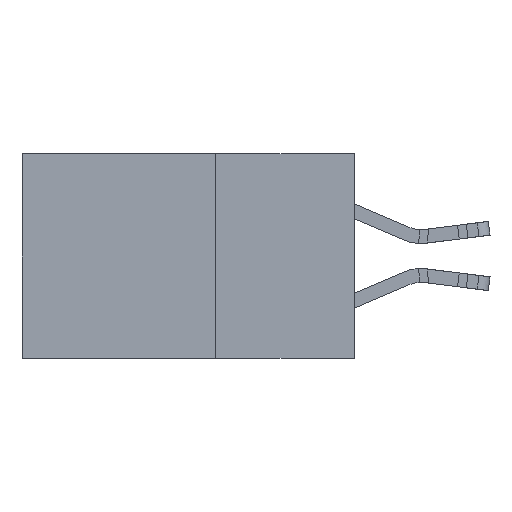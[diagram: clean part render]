
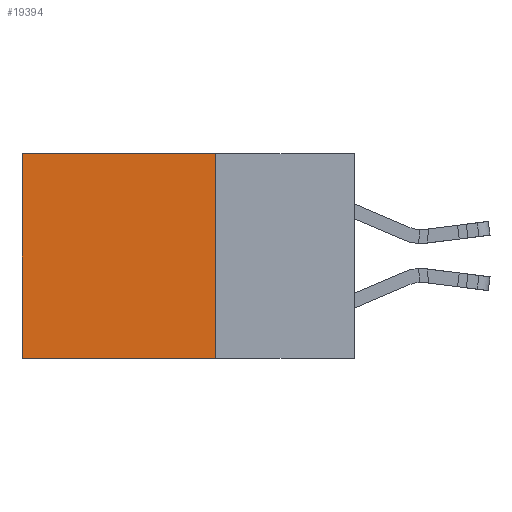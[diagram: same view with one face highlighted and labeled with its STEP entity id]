
A CAD part, left-side view. The second image highlights one B-rep face of the part: STEP entity #19394.
In plain terms, the highlighted planar face has unit normal (-1, 0, 0).
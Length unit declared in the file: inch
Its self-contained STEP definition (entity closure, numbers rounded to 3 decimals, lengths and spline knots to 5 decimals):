
#275 = LINE ( 'NONE', #14982, #15777 ) ;
#353 = ORIENTED_EDGE ( 'NONE', *, *, #2077, .T. ) ;
#1953 = ORIENTED_EDGE ( 'NONE', *, *, #19476, .F. ) ;
#2077 = EDGE_CURVE ( 'NONE', #3787, #19937, #25806, .T. ) ;
#2688 = CARTESIAN_POINT ( 'NONE',  ( 0.2615, 0.6, -0.37 ) ) ;
#3787 = VERTEX_POINT ( 'NONE', #11315 ) ;
#4360 = CARTESIAN_POINT ( 'NONE',  ( 0.2615, 0.25, 0. ) ) ;
#5278 = PLANE ( 'NONE',  #10027 ) ;
#6476 = CARTESIAN_POINT ( 'NONE',  ( 0.2615, 0.6, -0.37 ) ) ;
#6988 = ORIENTED_EDGE ( 'NONE', *, *, #23556, .F. ) ;
#7903 = DIRECTION ( 'NONE',  ( 0., 0., -1. ) ) ;
#8521 = DIRECTION ( 'NONE',  ( 0., 0., -1. ) ) ;
#10027 = AXIS2_PLACEMENT_3D ( 'NONE', #23342, #11432, #25301 ) ;
#10067 = VECTOR ( 'NONE', #21552, 39.37008 ) ;
#11315 = CARTESIAN_POINT ( 'NONE',  ( 0.2615, 0.6, 0. ) ) ;
#11432 = DIRECTION ( 'NONE',  ( 1., 0., 0. ) ) ;
#14345 = VERTEX_POINT ( 'NONE', #19765 ) ;
#14982 = CARTESIAN_POINT ( 'NONE',  ( 0.2615, 0.25, 0. ) ) ;
#15777 = VECTOR ( 'NONE', #24065, 39.37008 ) ;
#16615 = FACE_OUTER_BOUND ( 'NONE', #19851, .T. ) ;
#17083 = VECTOR ( 'NONE', #7903, 39.37008 ) ;
#17401 = EDGE_CURVE ( 'NONE', #19817, #3787, #275, .T. ) ;
#19394 = ADVANCED_FACE ( 'NONE', ( #16615 ), #5278, .F. ) ;
#19476 = EDGE_CURVE ( 'NONE', #14345, #19937, #25918, .T. ) ;
#19520 = CARTESIAN_POINT ( 'NONE',  ( 0.2615, 0.25, -0.37 ) ) ;
#19765 = CARTESIAN_POINT ( 'NONE',  ( 0.2615, 0.25, -0.37 ) ) ;
#19817 = VERTEX_POINT ( 'NONE', #4360 ) ;
#19851 = EDGE_LOOP ( 'NONE', ( #353, #1953, #6988, #19900 ) ) ;
#19900 = ORIENTED_EDGE ( 'NONE', *, *, #17401, .T. ) ;
#19937 = VERTEX_POINT ( 'NONE', #2688 ) ;
#21552 = DIRECTION ( 'NONE',  ( 0., 1., 0. ) ) ;
#21919 = CARTESIAN_POINT ( 'NONE',  ( 0.2615, 0.25, -0.37 ) ) ;
#23021 = LINE ( 'NONE', #21919, #17083 ) ;
#23342 = CARTESIAN_POINT ( 'NONE',  ( 0.2615, 0.25, -0.37 ) ) ;
#23556 = EDGE_CURVE ( 'NONE', #19817, #14345, #23021, .T. ) ;
#24065 = DIRECTION ( 'NONE',  ( 0., 1., 0. ) ) ;
#25199 = VECTOR ( 'NONE', #8521, 39.37008 ) ;
#25301 = DIRECTION ( 'NONE',  ( 0., 0., -1. ) ) ;
#25806 = LINE ( 'NONE', #6476, #25199 ) ;
#25918 = LINE ( 'NONE', #19520, #10067 ) ;
